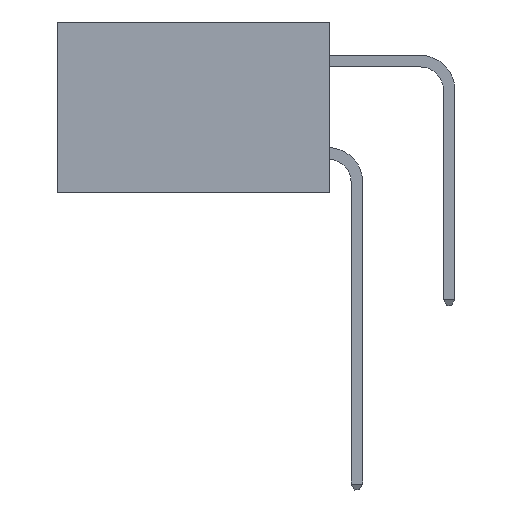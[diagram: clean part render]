
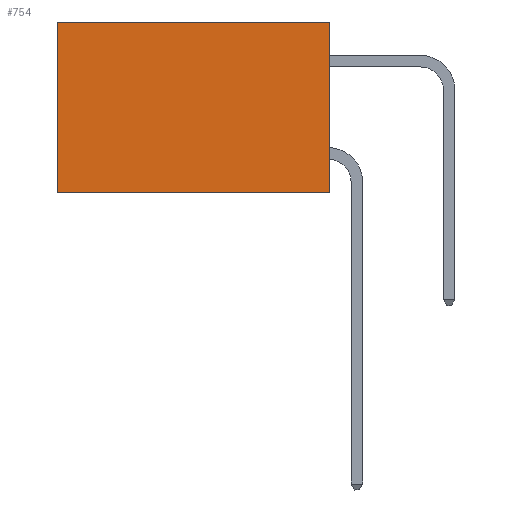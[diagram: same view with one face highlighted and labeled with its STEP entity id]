
A CAD part, left-side view. The second image highlights one B-rep face of the part: STEP entity #754.
In plain terms, the highlighted planar face has unit normal (-1, 0, 0).
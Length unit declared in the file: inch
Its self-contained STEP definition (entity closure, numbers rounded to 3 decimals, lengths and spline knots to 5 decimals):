
#658 = DIRECTION ( 'NONE',  ( 0., 0., -1. ) ) ;
#754 = ADVANCED_FACE ( 'NONE', ( #1351 ), #7292, .F. ) ;
#1349 = DIRECTION ( 'NONE',  ( 0., 0., -1. ) ) ;
#1351 = FACE_OUTER_BOUND ( 'NONE', #11769, .T. ) ;
#1371 = ORIENTED_EDGE ( 'NONE', *, *, #10492, .T. ) ;
#1622 = VECTOR ( 'NONE', #1349, 39.37008 ) ;
#1825 = VERTEX_POINT ( 'NONE', #9311 ) ;
#1935 = LINE ( 'NONE', #9075, #1622 ) ;
#2418 = AXIS2_PLACEMENT_3D ( 'NONE', #6232, #3257, #10754 ) ;
#3257 = DIRECTION ( 'NONE',  ( 1., 0., 0. ) ) ;
#3501 = CARTESIAN_POINT ( 'NONE',  ( 0.277, 0.59, 0. ) ) ;
#3645 = CARTESIAN_POINT ( 'NONE',  ( 0.277, 0.59, -0.37 ) ) ;
#3827 = LINE ( 'NONE', #3645, #6081 ) ;
#4673 = VECTOR ( 'NONE', #10320, 39.37008 ) ;
#4676 = VERTEX_POINT ( 'NONE', #12288 ) ;
#4831 = EDGE_CURVE ( 'NONE', #1825, #9943, #6869, .T. ) ;
#6081 = VECTOR ( 'NONE', #658, 39.37008 ) ;
#6232 = CARTESIAN_POINT ( 'NONE',  ( 0.277, 0., -0.37 ) ) ;
#6869 = LINE ( 'NONE', #10795, #4673 ) ;
#7292 = PLANE ( 'NONE',  #2418 ) ;
#7689 = CARTESIAN_POINT ( 'NONE',  ( 0.277, 0., 0. ) ) ;
#7975 = LINE ( 'NONE', #7689, #10216 ) ;
#8237 = EDGE_CURVE ( 'NONE', #4676, #1825, #1935, .T. ) ;
#8645 = DIRECTION ( 'NONE',  ( 0., 1., 0. ) ) ;
#9075 = CARTESIAN_POINT ( 'NONE',  ( 0.277, 0., -0.37 ) ) ;
#9215 = ORIENTED_EDGE ( 'NONE', *, *, #8237, .F. ) ;
#9311 = CARTESIAN_POINT ( 'NONE',  ( 0.277, 0., -0.37 ) ) ;
#9722 = EDGE_CURVE ( 'NONE', #10608, #9943, #3827, .T. ) ;
#9943 = VERTEX_POINT ( 'NONE', #12485 ) ;
#10216 = VECTOR ( 'NONE', #8645, 39.37008 ) ;
#10320 = DIRECTION ( 'NONE',  ( 0., 1., 0. ) ) ;
#10492 = EDGE_CURVE ( 'NONE', #4676, #10608, #7975, .T. ) ;
#10608 = VERTEX_POINT ( 'NONE', #3501 ) ;
#10754 = DIRECTION ( 'NONE',  ( 0., 0., -1. ) ) ;
#10795 = CARTESIAN_POINT ( 'NONE',  ( 0.277, 0., -0.37 ) ) ;
#11202 = ORIENTED_EDGE ( 'NONE', *, *, #9722, .T. ) ;
#11769 = EDGE_LOOP ( 'NONE', ( #11202, #12021, #9215, #1371 ) ) ;
#12021 = ORIENTED_EDGE ( 'NONE', *, *, #4831, .F. ) ;
#12288 = CARTESIAN_POINT ( 'NONE',  ( 0.277, 0., 0. ) ) ;
#12485 = CARTESIAN_POINT ( 'NONE',  ( 0.277, 0.59, -0.37 ) ) ;
